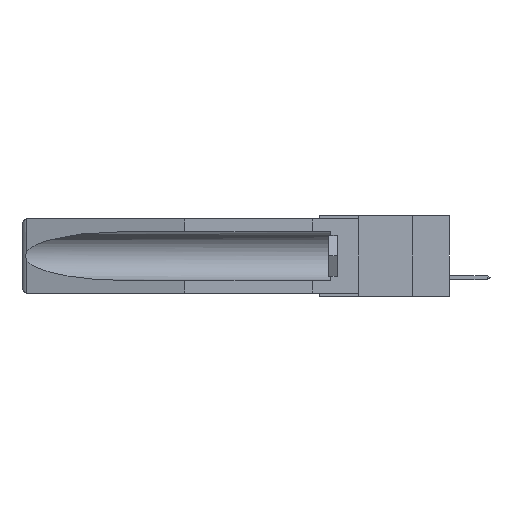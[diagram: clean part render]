
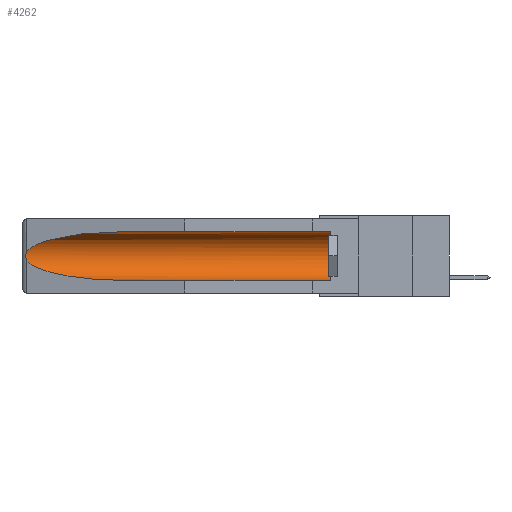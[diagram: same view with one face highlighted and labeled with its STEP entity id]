
A CAD part, left-side view. The second image highlights one B-rep face of the part: STEP entity #4262.
In plain terms, the highlighted cylindrical face has radius 2.857 mm (diameter 5.715 mm), a partial arc.
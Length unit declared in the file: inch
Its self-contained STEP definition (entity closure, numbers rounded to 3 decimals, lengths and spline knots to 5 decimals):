
#322 = CARTESIAN_POINT ( 'NONE',  ( 0.155, 0.126, -0.284 ) ) ;
#380 = CARTESIAN_POINT ( 'NONE',  ( 0.26537, 1.52718, -0.19328 ) ) ;
#504 = CARTESIAN_POINT ( 'NONE',  ( 0.26654, 1.53092, -0.15636 ) ) ;
#1884 = CARTESIAN_POINT ( 'NONE',  ( 0.155, 0.126, -0.1715 ) ) ;
#1897 = CARTESIAN_POINT ( 'NONE',  ( 0.2673, 1.5327, -0.16383 ) ) ;
#2083 = ORIENTED_EDGE ( 'NONE', *, *, #7651, .F. ) ;
#2223 = ORIENTED_EDGE ( 'NONE', *, *, #16619, .T. ) ;
#2431 =( BOUNDED_CURVE ( )  B_SPLINE_CURVE ( 3, ( #17398, #7750, #6285, #17275 ),
 .UNSPECIFIED., .F., .F. ) 
 B_SPLINE_CURVE_WITH_KNOTS ( ( 4, 4 ),
 ( 0.1948, 1.5708 ),
 .UNSPECIFIED. ) 
 CURVE ( )  GEOMETRIC_REPRESENTATION_ITEM ( )  RATIONAL_B_SPLINE_CURVE ( ( 1., 0.848, 0.848, 1. ) ) 
 REPRESENTATION_ITEM ( '' )  );
#2552 = DIRECTION ( 'NONE',  ( 0., 0., 1. ) ) ;
#2926 = CIRCLE ( 'NONE', #13741, 0.1125 ) ;
#3030 = CARTESIAN_POINT ( 'NONE',  ( 0.26537, 1.52718, -0.14972 ) ) ;
#3048 = VECTOR ( 'NONE', #9540, 39.37008 ) ;
#3216 = CARTESIAN_POINT ( 'NONE',  ( 0.2673, 1.53269, -0.17917 ) ) ;
#3340 = CARTESIAN_POINT ( 'NONE',  ( 0.2675, 1.53308, -0.17534 ) ) ;
#3369 = DIRECTION ( 'NONE',  ( 0., 1., 0. ) ) ;
#3558 = ORIENTED_EDGE ( 'NONE', *, *, #12296, .T. ) ;
#3847 = CARTESIAN_POINT ( 'NONE',  ( 0.155, -0.30754, -0.059 ) ) ;
#4262 = ADVANCED_FACE ( 'NONE', ( #6787 ), #10057, .F. ) ;
#4420 = CARTESIAN_POINT ( 'NONE',  ( 0.26597, 1.52961, -0.15275 ) ) ;
#4715 = CARTESIAN_POINT ( 'NONE',  ( 0.26597, 1.5296, -0.19026 ) ) ;
#5147 = ORIENTED_EDGE ( 'NONE', *, *, #15447, .T. ) ;
#5307 = VERTEX_POINT ( 'NONE', #9587 ) ;
#5645 = LINE ( 'NONE', #3847, #3048 ) ;
#5810 = CARTESIAN_POINT ( 'NONE',  ( 0.155, -0.30754, -0.1715 ) ) ;
#6285 = CARTESIAN_POINT ( 'NONE',  ( 0.21114, 1.30732, -0.284 ) ) ;
#6787 = FACE_OUTER_BOUND ( 'NONE', #10959, .T. ) ;
#7258 = CARTESIAN_POINT ( 'NONE',  ( 0.26655, 1.53094, -0.18657 ) ) ;
#7651 = EDGE_CURVE ( 'NONE', #13870, #14838, #12371, .T. ) ;
#7663 = CARTESIAN_POINT ( 'NONE',  ( 0.155, -0.30754, -0.284 ) ) ;
#7750 = CARTESIAN_POINT ( 'NONE',  ( 0.25451, 1.48313, -0.24835 ) ) ;
#7930 = CARTESIAN_POINT ( 'NONE',  ( 0.155, 1.07973, -0.059 ) ) ;
#7967 = CARTESIAN_POINT ( 'NONE',  ( 0.155, 1.07973, -0.059 ) ) ;
#8037 = ORIENTED_EDGE ( 'NONE', *, *, #10251, .T. ) ;
#8395 = AXIS2_PLACEMENT_3D ( 'NONE', #5810, #9514, #2552 ) ;
#8521 = VERTEX_POINT ( 'NONE', #7930 ) ;
#8542 = CARTESIAN_POINT ( 'NONE',  ( 0.26537, 1.52718, -0.19328 ) ) ;
#8733 = VERTEX_POINT ( 'NONE', #12645 ) ;
#9514 = DIRECTION ( 'NONE',  ( 0., 1., 0. ) ) ;
#9540 = DIRECTION ( 'NONE',  ( 0., 1., 0. ) ) ;
#9587 = CARTESIAN_POINT ( 'NONE',  ( 0.26537, 1.52718, -0.14972 ) ) ;
#10057 = CYLINDRICAL_SURFACE ( 'NONE', #8395, 0.1125 ) ;
#10251 = EDGE_CURVE ( 'NONE', #8521, #5307, #11664, .T. ) ;
#10846 = CARTESIAN_POINT ( 'NONE',  ( 0.21114, 1.30732, -0.059 ) ) ;
#10959 = EDGE_LOOP ( 'NONE', ( #8037, #11985, #2223, #2083, #3558, #5147 ) ) ;
#11664 =( BOUNDED_CURVE ( )  B_SPLINE_CURVE ( 3, ( #7967, #10846, #16299, #17807 ),
 .UNSPECIFIED., .F., .F. ) 
 B_SPLINE_CURVE_WITH_KNOTS ( ( 4, 4 ),
 ( 4.71239, 6.08839 ),
 .UNSPECIFIED. ) 
 CURVE ( )  GEOMETRIC_REPRESENTATION_ITEM ( )  RATIONAL_B_SPLINE_CURVE ( ( 1., 0.848, 0.848, 1. ) ) 
 REPRESENTATION_ITEM ( '' )  );
#11985 = ORIENTED_EDGE ( 'NONE', *, *, #13766, .T. ) ;
#12296 = EDGE_CURVE ( 'NONE', #13870, #8733, #2926, .T. ) ;
#12371 = LINE ( 'NONE', #7663, #15173 ) ;
#12645 = CARTESIAN_POINT ( 'NONE',  ( 0.155, 0.126, -0.059 ) ) ;
#13069 = DIRECTION ( 'NONE',  ( 0., 0., 1. ) ) ;
#13421 = CARTESIAN_POINT ( 'NONE',  ( 0.155, 1.07973, -0.284 ) ) ;
#13741 = AXIS2_PLACEMENT_3D ( 'NONE', #1884, #15894, #13069 ) ;
#13766 = EDGE_CURVE ( 'NONE', #5307, #14598, #16664, .T. ) ;
#13870 = VERTEX_POINT ( 'NONE', #322 ) ;
#14598 = VERTEX_POINT ( 'NONE', #8542 ) ;
#14838 = VERTEX_POINT ( 'NONE', #13421 ) ;
#15173 = VECTOR ( 'NONE', #3369, 39.37008 ) ;
#15447 = EDGE_CURVE ( 'NONE', #8733, #8521, #5645, .T. ) ;
#15787 = CARTESIAN_POINT ( 'NONE',  ( 0.2675, 1.53308, -0.16763 ) ) ;
#15894 = DIRECTION ( 'NONE',  ( 0., -1., 0. ) ) ;
#16299 = CARTESIAN_POINT ( 'NONE',  ( 0.25451, 1.48313, -0.09465 ) ) ;
#16619 = EDGE_CURVE ( 'NONE', #14598, #14838, #2431, .T. ) ;
#16664 = B_SPLINE_CURVE_WITH_KNOTS ( 'NONE', 3,
 ( #3030, #4420, #504, #1897, #15787, #3340, #3216, #7258, #4715, #380 ),
 .UNSPECIFIED., .F., .F.,
 ( 4, 2, 2, 2, 4 ),
 ( 0., 0.00029, 0.00058, 0.00087, 0.00117 ),
 .UNSPECIFIED. ) ;
#17275 = CARTESIAN_POINT ( 'NONE',  ( 0.155, 1.07973, -0.284 ) ) ;
#17398 = CARTESIAN_POINT ( 'NONE',  ( 0.26537, 1.52718, -0.19328 ) ) ;
#17807 = CARTESIAN_POINT ( 'NONE',  ( 0.26537, 1.52718, -0.14972 ) ) ;
